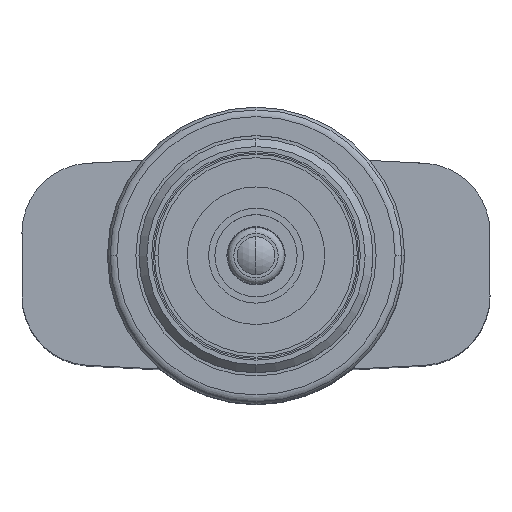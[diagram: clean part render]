
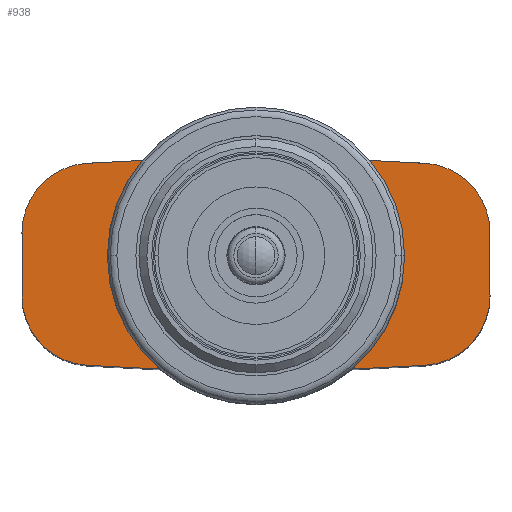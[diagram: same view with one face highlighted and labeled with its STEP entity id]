
A CAD part, top view. The second image highlights one B-rep face of the part: STEP entity #938.
In plain terms, the highlighted planar face has unit normal (0, 0, 1).
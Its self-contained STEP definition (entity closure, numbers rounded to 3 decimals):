
#62 = CARTESIAN_POINT ( 'NONE',  ( 45.369, 3.179, -151.788 ) ) ;
#63 = CARTESIAN_POINT ( 'NONE',  ( 45.2, -1.015, -151.788 ) ) ;
#75 = ORIENTED_EDGE ( 'NONE', *, *, #2695, .T. ) ;
#157 = AXIS2_PLACEMENT_3D ( 'NONE', #1903, #220, #596 ) ;
#191 = CARTESIAN_POINT ( 'NONE',  ( 34.631, -3.208, -151.788 ) ) ;
#203 = CARTESIAN_POINT ( 'NONE',  ( 47.4, -0.015, -151.788 ) ) ;
#218 = CARTESIAN_POINT ( 'NONE',  ( 40., 66.585, -151.788 ) ) ;
#220 = DIRECTION ( 'NONE',  ( 0., 0., -1. ) ) ;
#236 = CARTESIAN_POINT ( 'NONE',  ( 32.6, -1.015, -151.788 ) ) ;
#248 = VERTEX_POINT ( 'NONE', #3751 ) ;
#261 = DIRECTION ( 'NONE',  ( -1., 0., 0. ) ) ;
#281 = EDGE_CURVE ( 'NONE', #3930, #1450, #1161, .T. ) ;
#303 = CARTESIAN_POINT ( 'NONE',  ( 47.4, 0.986, -151.788 ) ) ;
#336 = ORIENTED_EDGE ( 'NONE', *, *, #3104, .F. ) ;
#390 = DIRECTION ( 'NONE',  ( 0., 0., 1. ) ) ;
#459 = DIRECTION ( 'NONE',  ( 0., 0., -1. ) ) ;
#555 = DIRECTION ( 'NONE',  ( 0., -1., 0. ) ) ;
#568 = VECTOR ( 'NONE', #555, 1000. ) ;
#592 = CARTESIAN_POINT ( 'NONE',  ( 32.6, 0.986, -151.788 ) ) ;
#596 = DIRECTION ( 'NONE',  ( -1., 0., 0. ) ) ;
#603 = EDGE_CURVE ( 'NONE', #2489, #1450, #2070, .T. ) ;
#624 = CARTESIAN_POINT ( 'NONE',  ( 42.75, -0.015, -151.788 ) ) ;
#787 = AXIS2_PLACEMENT_3D ( 'NONE', #63, #390, #1052 ) ;
#870 = FACE_OUTER_BOUND ( 'NONE', #3299, .T. ) ;
#938 = ADVANCED_FACE ( 'NONE', ( #870, #1526 ), #1571, .T. ) ;
#1052 = DIRECTION ( 'NONE',  ( -1., 0., 0. ) ) ;
#1080 = AXIS2_PLACEMENT_3D ( 'NONE', #4258, #3543, #261 ) ;
#1161 = LINE ( 'NONE', #3942, #568 ) ;
#1211 = EDGE_CURVE ( 'NONE', #1857, #2798, #4275, .T. ) ;
#1225 = CARTESIAN_POINT ( 'NONE',  ( 47.4, -1.015, -151.788 ) ) ;
#1228 = DIRECTION ( 'NONE',  ( 0., 1., 0. ) ) ;
#1261 = DIRECTION ( 'NONE',  ( 0., 0., 1. ) ) ;
#1268 = CARTESIAN_POINT ( 'NONE',  ( 45.364, -3.209, -151.788 ) ) ;
#1450 = VERTEX_POINT ( 'NONE', #236 ) ;
#1494 = AXIS2_PLACEMENT_3D ( 'NONE', #2280, #1944, #3223 ) ;
#1526 = FACE_BOUND ( 'NONE', #1612, .T. ) ;
#1556 = LINE ( 'NONE', #203, #3067 ) ;
#1571 = PLANE ( 'NONE',  #1080 ) ;
#1612 = EDGE_LOOP ( 'NONE', ( #2514, #4291 ) ) ;
#1703 = CARTESIAN_POINT ( 'NONE',  ( 34.8, 0.986, -151.788 ) ) ;
#1721 = CARTESIAN_POINT ( 'NONE',  ( 40., -0.015, -151.788 ) ) ;
#1805 = EDGE_CURVE ( 'NONE', #2798, #3886, #1556, .T. ) ;
#1817 = DIRECTION ( 'NONE',  ( -1., 0., 0. ) ) ;
#1857 = VERTEX_POINT ( 'NONE', #1268 ) ;
#1903 = CARTESIAN_POINT ( 'NONE',  ( 34.8, -1.015, -151.788 ) ) ;
#1944 = DIRECTION ( 'NONE',  ( 0., 0., 1. ) ) ;
#2043 = EDGE_CURVE ( 'NONE', #3528, #4259, #2635, .T. ) ;
#2070 = CIRCLE ( 'NONE', #157, 2.2 ) ;
#2191 = AXIS2_PLACEMENT_3D ( 'NONE', #4306, #1261, #4041 ) ;
#2192 = ORIENTED_EDGE ( 'NONE', *, *, #281, .T. ) ;
#2203 = AXIS2_PLACEMENT_3D ( 'NONE', #2852, #459, #1817 ) ;
#2227 = ORIENTED_EDGE ( 'NONE', *, *, #603, .F. ) ;
#2275 = CIRCLE ( 'NONE', #3752, 70. ) ;
#2280 = CARTESIAN_POINT ( 'NONE',  ( 45.2, 0.986, -151.788 ) ) ;
#2419 = EDGE_CURVE ( 'NONE', #4259, #3528, #3765, .T. ) ;
#2476 = EDGE_CURVE ( 'NONE', #3886, #3971, #3123, .T. ) ;
#2489 = VERTEX_POINT ( 'NONE', #191 ) ;
#2514 = ORIENTED_EDGE ( 'NONE', *, *, #2419, .T. ) ;
#2635 = CIRCLE ( 'NONE', #3555, 2.75 ) ;
#2695 = EDGE_CURVE ( 'NONE', #248, #3930, #3467, .T. ) ;
#2798 = VERTEX_POINT ( 'NONE', #1225 ) ;
#2845 = ORIENTED_EDGE ( 'NONE', *, *, #1211, .T. ) ;
#2852 = CARTESIAN_POINT ( 'NONE',  ( 40., -0.015, -151.788 ) ) ;
#2927 = ORIENTED_EDGE ( 'NONE', *, *, #2476, .T. ) ;
#2985 = CARTESIAN_POINT ( 'NONE',  ( 37.25, -0.015, -151.788 ) ) ;
#3047 = DIRECTION ( 'NONE',  ( 0., 0., 1. ) ) ;
#3064 = DIRECTION ( 'NONE',  ( 0., 0., -1. ) ) ;
#3067 = VECTOR ( 'NONE', #1228, 1000. ) ;
#3102 = DIRECTION ( 'NONE',  ( -1., 0., 0. ) ) ;
#3104 = EDGE_CURVE ( 'NONE', #1857, #2489, #2275, .T. ) ;
#3107 = CIRCLE ( 'NONE', #2191, 70. ) ;
#3123 = CIRCLE ( 'NONE', #1494, 2.2 ) ;
#3139 = EDGE_CURVE ( 'NONE', #3971, #248, #3107, .T. ) ;
#3223 = DIRECTION ( 'NONE',  ( -1., 0., 0. ) ) ;
#3273 = DIRECTION ( 'NONE',  ( -1., 0., 0. ) ) ;
#3299 = EDGE_LOOP ( 'NONE', ( #75, #2192, #2227, #336, #2845, #4301, #2927, #4274 ) ) ;
#3309 = DIRECTION ( 'NONE',  ( -1., 0., 0. ) ) ;
#3396 = AXIS2_PLACEMENT_3D ( 'NONE', #1703, #3047, #3309 ) ;
#3467 = CIRCLE ( 'NONE', #3396, 2.2 ) ;
#3528 = VERTEX_POINT ( 'NONE', #2985 ) ;
#3543 = DIRECTION ( 'NONE',  ( 0., 0., 1. ) ) ;
#3555 = AXIS2_PLACEMENT_3D ( 'NONE', #1721, #3064, #3102 ) ;
#3569 = DIRECTION ( 'NONE',  ( 0., 0., -1. ) ) ;
#3751 = CARTESIAN_POINT ( 'NONE',  ( 34.633, 3.179, -151.788 ) ) ;
#3752 = AXIS2_PLACEMENT_3D ( 'NONE', #218, #3569, #3273 ) ;
#3765 = CIRCLE ( 'NONE', #2203, 2.75 ) ;
#3886 = VERTEX_POINT ( 'NONE', #303 ) ;
#3930 = VERTEX_POINT ( 'NONE', #592 ) ;
#3942 = CARTESIAN_POINT ( 'NONE',  ( 32.6, -0.015, -151.788 ) ) ;
#3971 = VERTEX_POINT ( 'NONE', #62 ) ;
#4041 = DIRECTION ( 'NONE',  ( -1., 0., 0. ) ) ;
#4258 = CARTESIAN_POINT ( 'NONE',  ( 40., -0.015, -151.788 ) ) ;
#4259 = VERTEX_POINT ( 'NONE', #624 ) ;
#4274 = ORIENTED_EDGE ( 'NONE', *, *, #3139, .T. ) ;
#4275 = CIRCLE ( 'NONE', #787, 2.2 ) ;
#4291 = ORIENTED_EDGE ( 'NONE', *, *, #2043, .T. ) ;
#4301 = ORIENTED_EDGE ( 'NONE', *, *, #1805, .T. ) ;
#4306 = CARTESIAN_POINT ( 'NONE',  ( 40., -66.615, -151.788 ) ) ;
